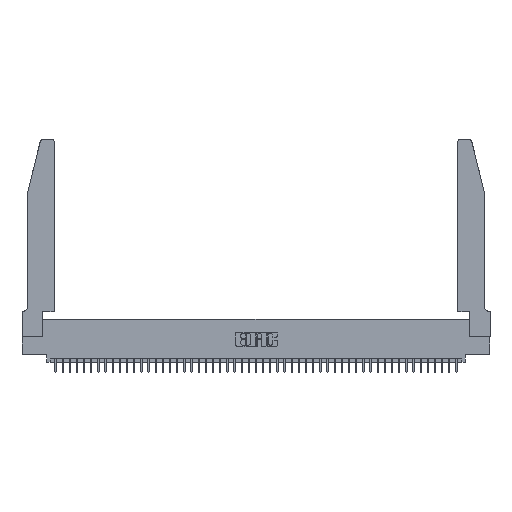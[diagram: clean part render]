
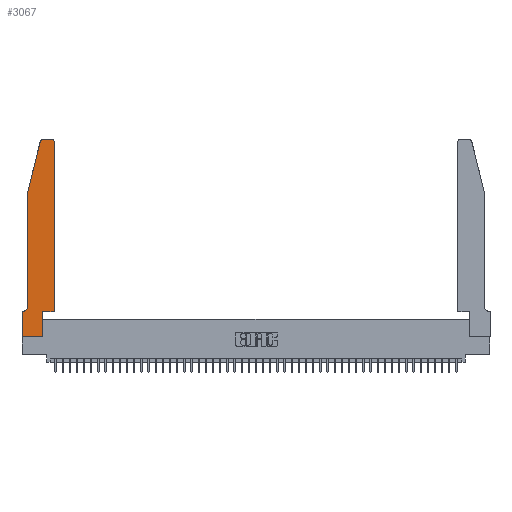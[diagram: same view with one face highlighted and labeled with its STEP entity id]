
A CAD part, top view. The second image highlights one B-rep face of the part: STEP entity #3067.
In plain terms, the highlighted planar face has unit normal (0, 0, 1).
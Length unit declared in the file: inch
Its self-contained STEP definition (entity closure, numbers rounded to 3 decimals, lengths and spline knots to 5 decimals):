
#270 = VECTOR ( 'NONE', #25938, 39.37008 ) ;
#303 = EDGE_CURVE ( 'NONE', #4009, #29886, #3934, .T. ) ;
#549 = EDGE_CURVE ( 'NONE', #8397, #27847, #24251, .T. ) ;
#1917 = CARTESIAN_POINT ( 'NONE',  ( 0.2865, 0., 0.37 ) ) ;
#2139 = ORIENTED_EDGE ( 'NONE', *, *, #27372, .T. ) ;
#2304 = CIRCLE ( 'NONE', #44716, 0.03 ) ;
#2399 = ORIENTED_EDGE ( 'NONE', *, *, #32243, .T. ) ;
#2667 = DIRECTION ( 'NONE',  ( 1., 0., 0. ) ) ;
#3067 = ADVANCED_FACE ( 'NONE', ( #47054 ), #22845, .T. ) ;
#3365 = CARTESIAN_POINT ( 'NONE',  ( 0.4505, 0.35, 0.37 ) ) ;
#3600 = CARTESIAN_POINT ( 'NONE',  ( 0.0755, 2., 0.37 ) ) ;
#3643 = LINE ( 'NONE', #10440, #18780 ) ;
#3934 = LINE ( 'NONE', #32957, #270 ) ;
#4009 = VERTEX_POINT ( 'NONE', #33121 ) ;
#6103 = EDGE_CURVE ( 'NONE', #6151, #46557, #2304, .T. ) ;
#6151 = VERTEX_POINT ( 'NONE', #31904 ) ;
#6180 = DIRECTION ( 'NONE',  ( 1., 0., 0. ) ) ;
#7350 = CARTESIAN_POINT ( 'NONE',  ( 0.0755, 2., 0.37 ) ) ;
#7878 = DIRECTION ( 'NONE',  ( 0., 1., 0. ) ) ;
#8397 = VERTEX_POINT ( 'NONE', #7350 ) ;
#8808 = CARTESIAN_POINT ( 'NONE',  ( 0., 0., 0.37 ) ) ;
#9140 = VECTOR ( 'NONE', #23687, 39.37008 ) ;
#9283 = VERTEX_POINT ( 'NONE', #13340 ) ;
#9311 = CARTESIAN_POINT ( 'NONE',  ( 0.284, 2.72, 0.37 ) ) ;
#10012 = CARTESIAN_POINT ( 'NONE',  ( 0.2865, 0.35, 0.37 ) ) ;
#10440 = CARTESIAN_POINT ( 'NONE',  ( 0.4505, 0.35, 0.37 ) ) ;
#11549 = EDGE_CURVE ( 'NONE', #22363, #47074, #3643, .T. ) ;
#11685 = DIRECTION ( 'NONE',  ( -1., 0., 0. ) ) ;
#12085 = AXIS2_PLACEMENT_3D ( 'NONE', #37590, #43667, #32587 ) ;
#12441 = CARTESIAN_POINT ( 'NONE',  ( 0., 0.35, 0.37 ) ) ;
#12479 = LINE ( 'NONE', #19486, #41059 ) ;
#13340 = CARTESIAN_POINT ( 'NONE',  ( 0.25487, 2.72718, 0.37 ) ) ;
#13940 = ORIENTED_EDGE ( 'NONE', *, *, #11549, .T. ) ;
#13952 = CARTESIAN_POINT ( 'NONE',  ( 0.2605, 2.75, 0.37 ) ) ;
#14649 = VERTEX_POINT ( 'NONE', #26198 ) ;
#15703 = CARTESIAN_POINT ( 'NONE',  ( 0., 0., 0.37 ) ) ;
#15990 = EDGE_CURVE ( 'NONE', #41975, #31109, #39814, .T. ) ;
#16198 = ORIENTED_EDGE ( 'NONE', *, *, #549, .T. ) ;
#16460 = CARTESIAN_POINT ( 'NONE',  ( 0.4205, 2.72, 0.37 ) ) ;
#17633 = ORIENTED_EDGE ( 'NONE', *, *, #41159, .T. ) ;
#18780 = VECTOR ( 'NONE', #33137, 39.37008 ) ;
#19217 = EDGE_LOOP ( 'NONE', ( #40122, #44002, #2139, #16198, #17633, #42086, #2399, #29881, #29333, #13940, #27844, #39521 ) ) ;
#19486 = CARTESIAN_POINT ( 'NONE',  ( 0.4505, 0.35, 0.37 ) ) ;
#19696 = EDGE_CURVE ( 'NONE', #46557, #14649, #29801, .T. ) ;
#21964 = VECTOR ( 'NONE', #46657, 39.37008 ) ;
#22168 = CARTESIAN_POINT ( 'NONE',  ( 0.0755, 0.42, 0.37 ) ) ;
#22180 = CARTESIAN_POINT ( 'NONE',  ( 0., 0., 0.37 ) ) ;
#22363 = VERTEX_POINT ( 'NONE', #10012 ) ;
#22736 = CIRCLE ( 'NONE', #35107, 0.07 ) ;
#22845 = PLANE ( 'NONE',  #12085 ) ;
#23214 = VECTOR ( 'NONE', #40318, 39.37008 ) ;
#23687 = DIRECTION ( 'NONE',  ( 0., -1., 0. ) ) ;
#24251 = LINE ( 'NONE', #28569, #21964 ) ;
#25938 = DIRECTION ( 'NONE',  ( -1., 0., 0. ) ) ;
#26198 = CARTESIAN_POINT ( 'NONE',  ( 0.284, 2.75, 0.37 ) ) ;
#26835 = EDGE_CURVE ( 'NONE', #14649, #9283, #40897, .T. ) ;
#27330 = VECTOR ( 'NONE', #28956, 39.37008 ) ;
#27372 = EDGE_CURVE ( 'NONE', #9283, #8397, #44178, .T. ) ;
#27844 = ORIENTED_EDGE ( 'NONE', *, *, #36568, .T. ) ;
#27847 = VERTEX_POINT ( 'NONE', #22168 ) ;
#27935 = CARTESIAN_POINT ( 'NONE',  ( 0.2865, 0.35, 0.37 ) ) ;
#28569 = CARTESIAN_POINT ( 'NONE',  ( 0.0755, 2., 0.37 ) ) ;
#28956 = DIRECTION ( 'NONE',  ( 1., 0., 0. ) ) ;
#29333 = ORIENTED_EDGE ( 'NONE', *, *, #37984, .T. ) ;
#29801 = LINE ( 'NONE', #13952, #35969 ) ;
#29881 = ORIENTED_EDGE ( 'NONE', *, *, #15990, .T. ) ;
#29886 = VERTEX_POINT ( 'NONE', #12441 ) ;
#30894 = AXIS2_PLACEMENT_3D ( 'NONE', #9311, #39272, #6180 ) ;
#31109 = VERTEX_POINT ( 'NONE', #1917 ) ;
#31192 = DIRECTION ( 'NONE',  ( 0., 0., 1. ) ) ;
#31904 = CARTESIAN_POINT ( 'NONE',  ( 0.4505, 2.72, 0.37 ) ) ;
#32243 = EDGE_CURVE ( 'NONE', #29886, #41975, #37943, .T. ) ;
#32259 = DIRECTION ( 'NONE',  ( 0., 1., 0. ) ) ;
#32587 = DIRECTION ( 'NONE',  ( 1., 0., 0. ) ) ;
#32957 = CARTESIAN_POINT ( 'NONE',  ( 0.0755, 0.35, 0.37 ) ) ;
#33121 = CARTESIAN_POINT ( 'NONE',  ( 0.0055, 0.35, 0.37 ) ) ;
#33137 = DIRECTION ( 'NONE',  ( 1., 0., 0. ) ) ;
#35045 = DIRECTION ( 'NONE',  ( -1., 0., 0. ) ) ;
#35107 = AXIS2_PLACEMENT_3D ( 'NONE', #35282, #42021, #35045 ) ;
#35282 = CARTESIAN_POINT ( 'NONE',  ( 0.0055, 0.42, 0.37 ) ) ;
#35969 = VECTOR ( 'NONE', #11685, 39.37008 ) ;
#36568 = EDGE_CURVE ( 'NONE', #47074, #6151, #12479, .T. ) ;
#37590 = CARTESIAN_POINT ( 'NONE',  ( 0., 0.35, 0.37 ) ) ;
#37943 = LINE ( 'NONE', #15703, #9140 ) ;
#37984 = EDGE_CURVE ( 'NONE', #31109, #22363, #46966, .T. ) ;
#39272 = DIRECTION ( 'NONE',  ( 0., 0., 1. ) ) ;
#39521 = ORIENTED_EDGE ( 'NONE', *, *, #6103, .T. ) ;
#39814 = LINE ( 'NONE', #22180, #27330 ) ;
#40122 = ORIENTED_EDGE ( 'NONE', *, *, #19696, .T. ) ;
#40318 = DIRECTION ( 'NONE',  ( -0.239, -0.971, 0. ) ) ;
#40897 = CIRCLE ( 'NONE', #30894, 0.03 ) ;
#41059 = VECTOR ( 'NONE', #7878, 39.37008 ) ;
#41159 = EDGE_CURVE ( 'NONE', #27847, #4009, #22736, .T. ) ;
#41975 = VERTEX_POINT ( 'NONE', #8808 ) ;
#42021 = DIRECTION ( 'NONE',  ( 0., 0., -1. ) ) ;
#42086 = ORIENTED_EDGE ( 'NONE', *, *, #303, .T. ) ;
#42591 = VECTOR ( 'NONE', #32259, 39.37008 ) ;
#43667 = DIRECTION ( 'NONE',  ( 0., 0., 1. ) ) ;
#44002 = ORIENTED_EDGE ( 'NONE', *, *, #26835, .T. ) ;
#44178 = LINE ( 'NONE', #3600, #23214 ) ;
#44716 = AXIS2_PLACEMENT_3D ( 'NONE', #16460, #31192, #2667 ) ;
#46557 = VERTEX_POINT ( 'NONE', #46903 ) ;
#46657 = DIRECTION ( 'NONE',  ( 0., -1., 0. ) ) ;
#46903 = CARTESIAN_POINT ( 'NONE',  ( 0.4205, 2.75, 0.37 ) ) ;
#46966 = LINE ( 'NONE', #27935, #42591 ) ;
#47054 = FACE_OUTER_BOUND ( 'NONE', #19217, .T. ) ;
#47074 = VERTEX_POINT ( 'NONE', #3365 ) ;
